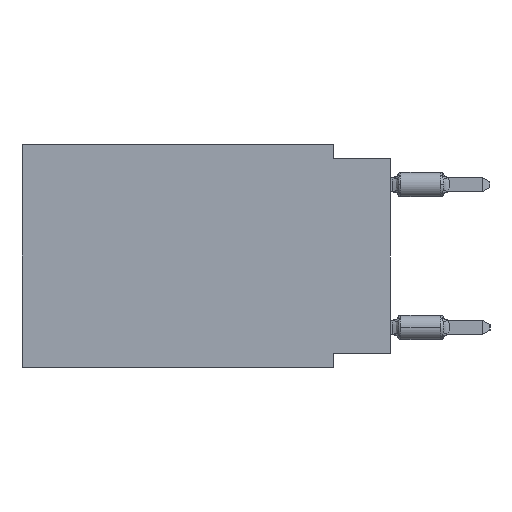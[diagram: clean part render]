
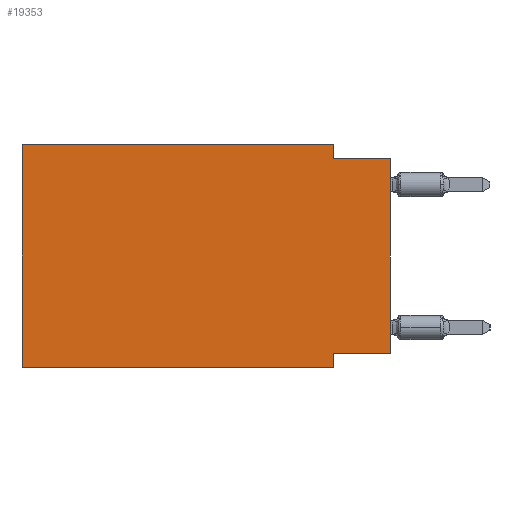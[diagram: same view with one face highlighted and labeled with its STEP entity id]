
A CAD part, left-side view. The second image highlights one B-rep face of the part: STEP entity #19353.
In plain terms, the highlighted planar face has unit normal (-1, 0, 0).
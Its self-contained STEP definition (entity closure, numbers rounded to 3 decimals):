
#172 = DIRECTION ( 'NONE',  ( 0., -1., 0. ) ) ;
#228 = DIRECTION ( 'NONE',  ( 0., -1., 0. ) ) ;
#334 = ORIENTED_EDGE ( 'NONE', *, *, #20344, .F. ) ;
#1336 = CARTESIAN_POINT ( 'NONE',  ( 0., 0., -9.271 ) ) ;
#1350 = VERTEX_POINT ( 'NONE', #12911 ) ;
#1461 = LINE ( 'NONE', #16188, #17121 ) ;
#1552 = VECTOR ( 'NONE', #13248, 1000. ) ;
#2333 = VECTOR ( 'NONE', #228, 1000. ) ;
#2706 = VECTOR ( 'NONE', #9415, 1000. ) ;
#2929 = VECTOR ( 'NONE', #172, 1000. ) ;
#3029 = DIRECTION ( 'NONE',  ( 0., -1., 0. ) ) ;
#3085 = DIRECTION ( 'NONE',  ( 1., 0., 0. ) ) ;
#3300 = LINE ( 'NONE', #7640, #1552 ) ;
#3958 = LINE ( 'NONE', #18445, #2929 ) ;
#4517 = CARTESIAN_POINT ( 'NONE',  ( 0., 0., -0.635 ) ) ;
#5422 = VERTEX_POINT ( 'NONE', #18160 ) ;
#5481 = VECTOR ( 'NONE', #9780, 1000. ) ;
#6440 = EDGE_CURVE ( 'NONE', #1350, #13760, #13655, .T. ) ;
#6441 = CARTESIAN_POINT ( 'NONE',  ( 0., 16.383, -9.906 ) ) ;
#6466 = CARTESIAN_POINT ( 'NONE',  ( 0., 16.383, 0. ) ) ;
#7306 = FACE_OUTER_BOUND ( 'NONE', #25821, .T. ) ;
#7432 = CARTESIAN_POINT ( 'NONE',  ( 0., 16.383, 0. ) ) ;
#7467 = EDGE_CURVE ( 'NONE', #20977, #25991, #1461, .T. ) ;
#7640 = CARTESIAN_POINT ( 'NONE',  ( 0., 16.383, 0. ) ) ;
#7719 = CARTESIAN_POINT ( 'NONE',  ( 0., 2.54, -0.635 ) ) ;
#9355 = PLANE ( 'NONE',  #14555 ) ;
#9415 = DIRECTION ( 'NONE',  ( 0., 0., -1. ) ) ;
#9606 = DIRECTION ( 'NONE',  ( 0., 0., -1. ) ) ;
#9780 = DIRECTION ( 'NONE',  ( 0., 0., 1. ) ) ;
#9938 = ORIENTED_EDGE ( 'NONE', *, *, #10657, .T. ) ;
#10036 = CARTESIAN_POINT ( 'NONE',  ( 0., 0., 0. ) ) ;
#10504 = ORIENTED_EDGE ( 'NONE', *, *, #15768, .F. ) ;
#10657 = EDGE_CURVE ( 'NONE', #13257, #25991, #25172, .T. ) ;
#11564 = ORIENTED_EDGE ( 'NONE', *, *, #12524, .F. ) ;
#12524 = EDGE_CURVE ( 'NONE', #21409, #20977, #20298, .T. ) ;
#12911 = CARTESIAN_POINT ( 'NONE',  ( 0., 2.54, 0. ) ) ;
#13248 = DIRECTION ( 'NONE',  ( 0., 0., 1. ) ) ;
#13257 = VERTEX_POINT ( 'NONE', #21439 ) ;
#13655 = LINE ( 'NONE', #24196, #2706 ) ;
#13760 = VERTEX_POINT ( 'NONE', #7719 ) ;
#13987 = DIRECTION ( 'NONE',  ( 0., 0., -1. ) ) ;
#14555 = AXIS2_PLACEMENT_3D ( 'NONE', #7432, #3085, #13987 ) ;
#15534 = VECTOR ( 'NONE', #26175, 1000. ) ;
#15768 = EDGE_CURVE ( 'NONE', #13760, #25153, #3958, .T. ) ;
#15886 = VECTOR ( 'NONE', #3029, 1000. ) ;
#16188 = CARTESIAN_POINT ( 'NONE',  ( 0., 2.54, -9.906 ) ) ;
#17121 = VECTOR ( 'NONE', #9606, 1000. ) ;
#17988 = EDGE_CURVE ( 'NONE', #5422, #1350, #21240, .T. ) ;
#18160 = CARTESIAN_POINT ( 'NONE',  ( 0., 16.383, 0. ) ) ;
#18445 = CARTESIAN_POINT ( 'NONE',  ( 0., 0., -0.635 ) ) ;
#18539 = CARTESIAN_POINT ( 'NONE',  ( 0., 2.54, -9.271 ) ) ;
#19353 = ADVANCED_FACE ( 'NONE', ( #7306 ), #9355, .F. ) ;
#20298 = LINE ( 'NONE', #1336, #15534 ) ;
#20344 = EDGE_CURVE ( 'NONE', #13257, #5422, #3300, .T. ) ;
#20934 = EDGE_CURVE ( 'NONE', #21409, #25153, #26605, .T. ) ;
#20977 = VERTEX_POINT ( 'NONE', #18539 ) ;
#21240 = LINE ( 'NONE', #6466, #2333 ) ;
#21409 = VERTEX_POINT ( 'NONE', #22217 ) ;
#21439 = CARTESIAN_POINT ( 'NONE',  ( 0., 16.383, -9.906 ) ) ;
#22217 = CARTESIAN_POINT ( 'NONE',  ( 0., 0., -9.271 ) ) ;
#23357 = ORIENTED_EDGE ( 'NONE', *, *, #7467, .F. ) ;
#24196 = CARTESIAN_POINT ( 'NONE',  ( 0., 2.54, 0. ) ) ;
#25101 = CARTESIAN_POINT ( 'NONE',  ( 0., 2.54, -9.906 ) ) ;
#25153 = VERTEX_POINT ( 'NONE', #4517 ) ;
#25172 = LINE ( 'NONE', #6441, #15886 ) ;
#25254 = ORIENTED_EDGE ( 'NONE', *, *, #20934, .T. ) ;
#25821 = EDGE_LOOP ( 'NONE', ( #25254, #10504, #26123, #26287, #334, #9938, #23357, #11564 ) ) ;
#25991 = VERTEX_POINT ( 'NONE', #25101 ) ;
#26123 = ORIENTED_EDGE ( 'NONE', *, *, #6440, .F. ) ;
#26175 = DIRECTION ( 'NONE',  ( 0., 1., 0. ) ) ;
#26287 = ORIENTED_EDGE ( 'NONE', *, *, #17988, .F. ) ;
#26605 = LINE ( 'NONE', #10036, #5481 ) ;
